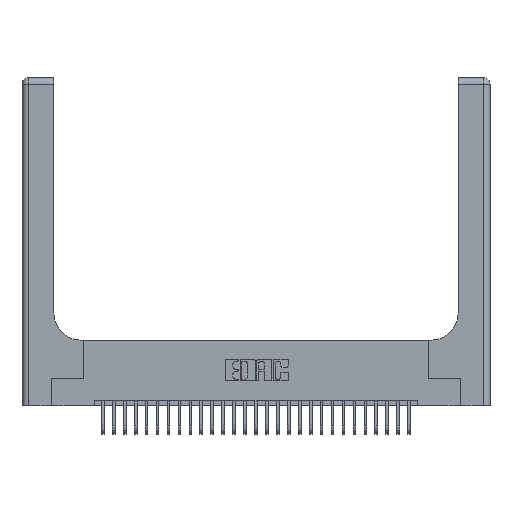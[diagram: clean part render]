
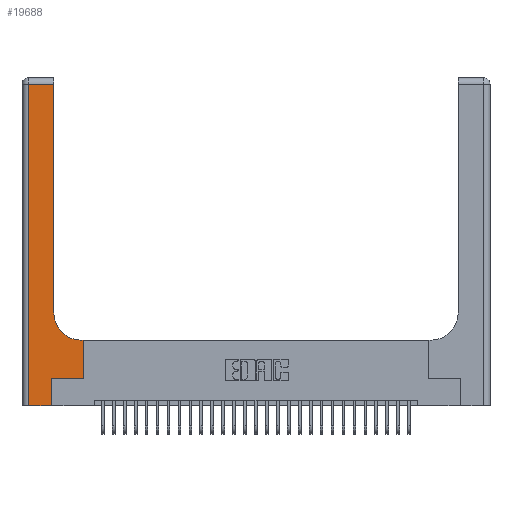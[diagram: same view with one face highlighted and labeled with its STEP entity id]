
A CAD part, top view. The second image highlights one B-rep face of the part: STEP entity #19688.
In plain terms, the highlighted planar face has unit normal (0, 0, 1).
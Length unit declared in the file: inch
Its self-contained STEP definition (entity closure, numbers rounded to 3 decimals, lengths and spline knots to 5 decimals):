
#189 = DIRECTION ( 'NONE',  ( 1., 0., 0. ) ) ;
#565 = ORIENTED_EDGE ( 'NONE', *, *, #5120, .T. ) ;
#870 = LINE ( 'NONE', #23042, #18967 ) ;
#1631 = PLANE ( 'NONE',  #7134 ) ;
#1748 = CARTESIAN_POINT ( 'NONE',  ( 0.269, 0.25, 0.37 ) ) ;
#1791 = ORIENTED_EDGE ( 'NONE', *, *, #4909, .T. ) ;
#1814 = CIRCLE ( 'NONE', #18620, 0.25 ) ;
#1911 = ORIENTED_EDGE ( 'NONE', *, *, #18407, .T. ) ;
#3248 = VECTOR ( 'NONE', #189, 39.37008 ) ;
#3349 = LINE ( 'NONE', #8773, #28771 ) ;
#3505 = VECTOR ( 'NONE', #6355, 39.37008 ) ;
#3895 = CARTESIAN_POINT ( 'NONE',  ( 0.269, 0., 0.37 ) ) ;
#4062 = DIRECTION ( 'NONE',  ( 0., 0., -1. ) ) ;
#4909 = EDGE_CURVE ( 'NONE', #15669, #19892, #3349, .T. ) ;
#5070 = CARTESIAN_POINT ( 'NONE',  ( 0.269, 0.25, 0.37 ) ) ;
#5120 = EDGE_CURVE ( 'NONE', #25896, #27761, #7142, .T. ) ;
#5740 = ORIENTED_EDGE ( 'NONE', *, *, #12844, .T. ) ;
#6355 = DIRECTION ( 'NONE',  ( 0., 1., 0. ) ) ;
#7134 = AXIS2_PLACEMENT_3D ( 'NONE', #30645, #4062, #16219 ) ;
#7142 = LINE ( 'NONE', #8330, #24905 ) ;
#7719 = CARTESIAN_POINT ( 'NONE',  ( 0.5585, 0.6, 0.37 ) ) ;
#8330 = CARTESIAN_POINT ( 'NONE',  ( 0.2915, 3., 0.37 ) ) ;
#8628 = CARTESIAN_POINT ( 'NONE',  ( 0.5415, 0.85, 0.37 ) ) ;
#8773 = CARTESIAN_POINT ( 'NONE',  ( 0.2915, 0.6, 0.37 ) ) ;
#8783 = DIRECTION ( 'NONE',  ( 0., -1., 0. ) ) ;
#9088 = CARTESIAN_POINT ( 'NONE',  ( 0.2915, 0.85, 0.37 ) ) ;
#9432 = ORIENTED_EDGE ( 'NONE', *, *, #16278, .T. ) ;
#9713 = LINE ( 'NONE', #12273, #3248 ) ;
#9772 = EDGE_CURVE ( 'NONE', #30126, #15669, #18202, .T. ) ;
#9837 = CARTESIAN_POINT ( 'NONE',  ( 0., 2.94, 0.37 ) ) ;
#10885 = DIRECTION ( 'NONE',  ( 0., 1., 0. ) ) ;
#11118 = VERTEX_POINT ( 'NONE', #19099 ) ;
#11192 = DIRECTION ( 'NONE',  ( 0., 0., -1. ) ) ;
#11980 = ORIENTED_EDGE ( 'NONE', *, *, #12980, .T. ) ;
#12173 = FACE_OUTER_BOUND ( 'NONE', #22054, .T. ) ;
#12273 = CARTESIAN_POINT ( 'NONE',  ( 0., 0., 0.37 ) ) ;
#12844 = EDGE_CURVE ( 'NONE', #27761, #24492, #24143, .T. ) ;
#12980 = EDGE_CURVE ( 'NONE', #19892, #25896, #1814, .T. ) ;
#15176 = VERTEX_POINT ( 'NONE', #28756 ) ;
#15669 = VERTEX_POINT ( 'NONE', #7719 ) ;
#16219 = DIRECTION ( 'NONE',  ( -1., 0., 0. ) ) ;
#16278 = EDGE_CURVE ( 'NONE', #15176, #11118, #9713, .T. ) ;
#16983 = CARTESIAN_POINT ( 'NONE',  ( 0.2915, 2.94, 0.37 ) ) ;
#18202 = LINE ( 'NONE', #28510, #28882 ) ;
#18407 = EDGE_CURVE ( 'NONE', #24492, #15176, #870, .T. ) ;
#18620 = AXIS2_PLACEMENT_3D ( 'NONE', #8628, #11192, #25463 ) ;
#18967 = VECTOR ( 'NONE', #8783, 39.37008 ) ;
#19099 = CARTESIAN_POINT ( 'NONE',  ( 0.269, 0., 0.37 ) ) ;
#19183 = CARTESIAN_POINT ( 'NONE',  ( 0.5585, 0.25, 0.37 ) ) ;
#19688 = ADVANCED_FACE ( 'NONE', ( #12173 ), #1631, .F. ) ;
#19892 = VERTEX_POINT ( 'NONE', #26396 ) ;
#20110 = LINE ( 'NONE', #1748, #22422 ) ;
#20869 = DIRECTION ( 'NONE',  ( 1., 0., 0. ) ) ;
#20915 = DIRECTION ( 'NONE',  ( -1., 0., 0. ) ) ;
#21889 = DIRECTION ( 'NONE',  ( 0., 1., 0. ) ) ;
#22054 = EDGE_LOOP ( 'NONE', ( #565, #5740, #1911, #9432, #25447, #23912, #24718, #1791, #11980 ) ) ;
#22422 = VECTOR ( 'NONE', #20869, 39.37008 ) ;
#22833 = EDGE_CURVE ( 'NONE', #11118, #25115, #27396, .T. ) ;
#23042 = CARTESIAN_POINT ( 'NONE',  ( 0.06, 3., 0.37 ) ) ;
#23377 = VECTOR ( 'NONE', #27715, 39.37008 ) ;
#23912 = ORIENTED_EDGE ( 'NONE', *, *, #30677, .T. ) ;
#24143 = LINE ( 'NONE', #9837, #23377 ) ;
#24492 = VERTEX_POINT ( 'NONE', #29782 ) ;
#24718 = ORIENTED_EDGE ( 'NONE', *, *, #9772, .T. ) ;
#24905 = VECTOR ( 'NONE', #10885, 39.37008 ) ;
#25115 = VERTEX_POINT ( 'NONE', #5070 ) ;
#25447 = ORIENTED_EDGE ( 'NONE', *, *, #22833, .T. ) ;
#25463 = DIRECTION ( 'NONE',  ( 1., 0., 0. ) ) ;
#25896 = VERTEX_POINT ( 'NONE', #9088 ) ;
#26396 = CARTESIAN_POINT ( 'NONE',  ( 0.5415, 0.6, 0.37 ) ) ;
#27396 = LINE ( 'NONE', #3895, #3505 ) ;
#27715 = DIRECTION ( 'NONE',  ( -1., 0., 0. ) ) ;
#27761 = VERTEX_POINT ( 'NONE', #16983 ) ;
#28510 = CARTESIAN_POINT ( 'NONE',  ( 0.5585, 0.25, 0.37 ) ) ;
#28756 = CARTESIAN_POINT ( 'NONE',  ( 0.06, 0., 0.37 ) ) ;
#28771 = VECTOR ( 'NONE', #20915, 39.37008 ) ;
#28882 = VECTOR ( 'NONE', #21889, 39.37008 ) ;
#29782 = CARTESIAN_POINT ( 'NONE',  ( 0.06, 2.94, 0.37 ) ) ;
#30126 = VERTEX_POINT ( 'NONE', #19183 ) ;
#30645 = CARTESIAN_POINT ( 'NONE',  ( 0., 3., 0.37 ) ) ;
#30677 = EDGE_CURVE ( 'NONE', #25115, #30126, #20110, .T. ) ;
